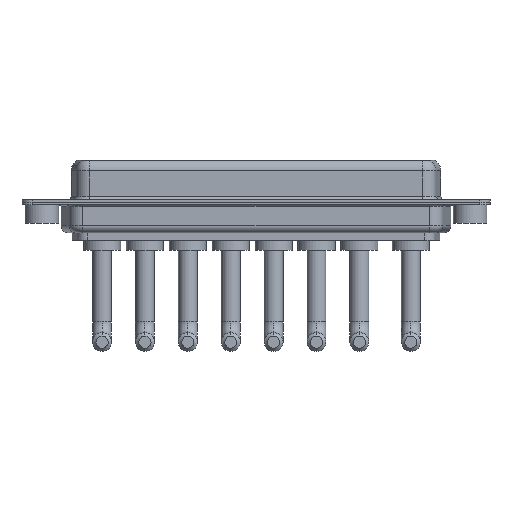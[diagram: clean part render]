
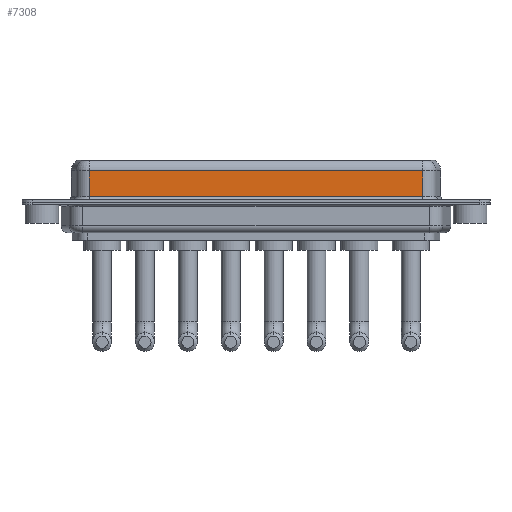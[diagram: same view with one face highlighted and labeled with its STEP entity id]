
A CAD part, front view. The second image highlights one B-rep face of the part: STEP entity #7308.
In plain terms, the highlighted planar face has unit normal (0, -1, 0).
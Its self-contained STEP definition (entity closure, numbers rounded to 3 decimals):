
#270 = LINE ( 'NONE', #7294, #4596 ) ;
#1941 = EDGE_CURVE ( 'NONE', #9611, #9208, #7991, .T. ) ;
#2268 = DIRECTION ( 'NONE',  ( 0., 1., 0. ) ) ;
#2563 = LINE ( 'NONE', #9880, #7460 ) ;
#2698 = DIRECTION ( 'NONE',  ( 0., 0., -1. ) ) ;
#2786 = CARTESIAN_POINT ( 'NONE',  ( 7.038, -3.95, 6.4 ) ) ;
#3071 = LINE ( 'NONE', #2786, #11358 ) ;
#4298 = PLANE ( 'NONE',  #9408 ) ;
#4351 = CARTESIAN_POINT ( 'NONE',  ( 7.038, -3.95, 4.65 ) ) ;
#4596 = VECTOR ( 'NONE', #11403, 1000. ) ;
#5359 = ORIENTED_EDGE ( 'NONE', *, *, #1941, .T. ) ;
#5387 = EDGE_CURVE ( 'NONE', #7448, #6609, #270, .T. ) ;
#6409 = CARTESIAN_POINT ( 'NONE',  ( 56.462, -3.95, 6.4 ) ) ;
#6609 = VERTEX_POINT ( 'NONE', #6969 ) ;
#6930 = DIRECTION ( 'NONE',  ( 0., 0., -1. ) ) ;
#6969 = CARTESIAN_POINT ( 'NONE',  ( 56.462, -3.95, 0.9 ) ) ;
#7174 = EDGE_LOOP ( 'NONE', ( #8910, #5359, #10021, #7941 ) ) ;
#7294 = CARTESIAN_POINT ( 'NONE',  ( 56.462, -3.95, 0.9 ) ) ;
#7308 = ADVANCED_FACE ( 'NONE', ( #9301 ), #4298, .F. ) ;
#7448 = VERTEX_POINT ( 'NONE', #11854 ) ;
#7460 = VECTOR ( 'NONE', #2698, 1000. ) ;
#7722 = EDGE_CURVE ( 'NONE', #9208, #7448, #3071, .T. ) ;
#7924 = DIRECTION ( 'NONE',  ( -1., 0., 0. ) ) ;
#7941 = ORIENTED_EDGE ( 'NONE', *, *, #5387, .T. ) ;
#7991 = LINE ( 'NONE', #13053, #8219 ) ;
#8219 = VECTOR ( 'NONE', #7924, 1000. ) ;
#8910 = ORIENTED_EDGE ( 'NONE', *, *, #11384, .F. ) ;
#9208 = VERTEX_POINT ( 'NONE', #4351 ) ;
#9301 = FACE_OUTER_BOUND ( 'NONE', #7174, .T. ) ;
#9408 = AXIS2_PLACEMENT_3D ( 'NONE', #6409, #2268, #9494 ) ;
#9494 = DIRECTION ( 'NONE',  ( 0., 0., 1. ) ) ;
#9611 = VERTEX_POINT ( 'NONE', #10216 ) ;
#9880 = CARTESIAN_POINT ( 'NONE',  ( 56.462, -3.95, 6.4 ) ) ;
#10021 = ORIENTED_EDGE ( 'NONE', *, *, #7722, .T. ) ;
#10216 = CARTESIAN_POINT ( 'NONE',  ( 56.462, -3.95, 4.65 ) ) ;
#11358 = VECTOR ( 'NONE', #6930, 1000. ) ;
#11384 = EDGE_CURVE ( 'NONE', #9611, #6609, #2563, .T. ) ;
#11403 = DIRECTION ( 'NONE',  ( 1., 0., 0. ) ) ;
#11854 = CARTESIAN_POINT ( 'NONE',  ( 7.038, -3.95, 0.9 ) ) ;
#13053 = CARTESIAN_POINT ( 'NONE',  ( 56.462, -3.95, 4.65 ) ) ;
